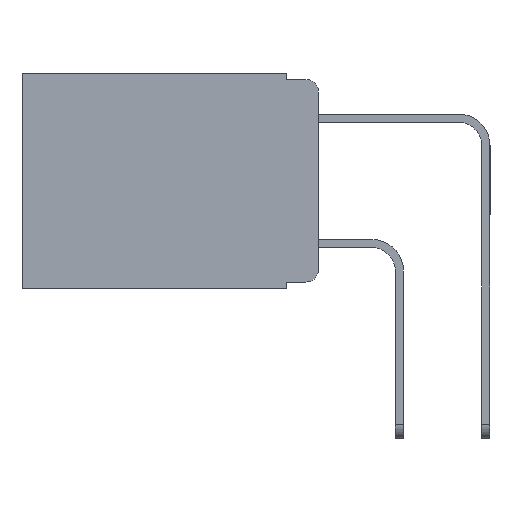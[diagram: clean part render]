
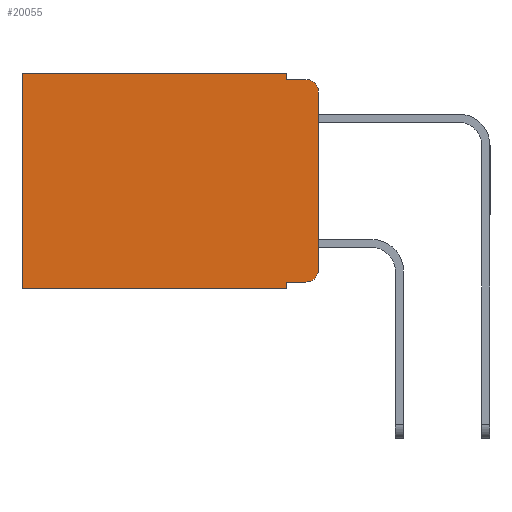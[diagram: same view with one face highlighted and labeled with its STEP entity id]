
A CAD part, left-side view. The second image highlights one B-rep face of the part: STEP entity #20055.
In plain terms, the highlighted planar face has unit normal (-1, 0, 0).
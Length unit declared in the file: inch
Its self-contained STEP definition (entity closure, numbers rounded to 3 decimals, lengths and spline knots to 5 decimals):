
#54 = CARTESIAN_POINT ( 'NONE',  ( 0.298, 0.051, -0.343 ) ) ;
#188 = LINE ( 'NONE', #1957, #16687 ) ;
#774 = AXIS2_PLACEMENT_3D ( 'NONE', #19364, #19434, #10102 ) ;
#894 = LINE ( 'NONE', #9400, #4678 ) ;
#959 = CARTESIAN_POINT ( 'NONE',  ( 0.298, 0.02, -0.313 ) ) ;
#1006 = VERTEX_POINT ( 'NONE', #2538 ) ;
#1144 = CARTESIAN_POINT ( 'NONE',  ( 0.298, 0., -0.03 ) ) ;
#1451 = CARTESIAN_POINT ( 'NONE',  ( 0.298, 0.051, -0.01 ) ) ;
#1523 = LINE ( 'NONE', #11746, #13294 ) ;
#1579 = EDGE_CURVE ( 'NONE', #17158, #1006, #1523, .T. ) ;
#1843 = ORIENTED_EDGE ( 'NONE', *, *, #18049, .F. ) ;
#1889 = LINE ( 'NONE', #14975, #10438 ) ;
#1957 = CARTESIAN_POINT ( 'NONE',  ( 0.298, 0., 0. ) ) ;
#2538 = CARTESIAN_POINT ( 'NONE',  ( 0.298, 0.473, -0.343 ) ) ;
#2570 = DIRECTION ( 'NONE',  ( 0., 0., -1. ) ) ;
#2742 = EDGE_CURVE ( 'NONE', #5668, #14277, #188, .T. ) ;
#3041 = CARTESIAN_POINT ( 'NONE',  ( 0.298, 0.02, -0.333 ) ) ;
#3396 = CARTESIAN_POINT ( 'NONE',  ( 0.298, 0.02, -0.03 ) ) ;
#3581 = CIRCLE ( 'NONE', #18429, 0.02 ) ;
#3601 = CIRCLE ( 'NONE', #11106, 0.02 ) ;
#3774 = VERTEX_POINT ( 'NONE', #10031 ) ;
#3812 = EDGE_CURVE ( 'NONE', #5950, #5194, #19744, .T. ) ;
#3840 = DIRECTION ( 'NONE',  ( 0., -1., 0. ) ) ;
#4229 = LINE ( 'NONE', #10632, #11732 ) ;
#4421 = DIRECTION ( 'NONE',  ( 0., -1., 0. ) ) ;
#4612 = ORIENTED_EDGE ( 'NONE', *, *, #2742, .F. ) ;
#4678 = VECTOR ( 'NONE', #18772, 39.37008 ) ;
#4864 = DIRECTION ( 'NONE',  ( 0., 0., -1. ) ) ;
#5055 = DIRECTION ( 'NONE',  ( 0., 0., -1. ) ) ;
#5194 = VERTEX_POINT ( 'NONE', #1451 ) ;
#5204 = VERTEX_POINT ( 'NONE', #12632 ) ;
#5668 = VERTEX_POINT ( 'NONE', #1144 ) ;
#5950 = VERTEX_POINT ( 'NONE', #6714 ) ;
#6148 = ORIENTED_EDGE ( 'NONE', *, *, #16682, .F. ) ;
#6321 = EDGE_CURVE ( 'NONE', #5194, #3774, #11871, .T. ) ;
#6486 = CARTESIAN_POINT ( 'NONE',  ( 0.298, 0.051, 0. ) ) ;
#6655 = ORIENTED_EDGE ( 'NONE', *, *, #18412, .T. ) ;
#6714 = CARTESIAN_POINT ( 'NONE',  ( 0.298, 0.051, 0. ) ) ;
#7264 = DIRECTION ( 'NONE',  ( 0., 0., -1. ) ) ;
#7406 = VECTOR ( 'NONE', #4864, 39.37008 ) ;
#7438 = CARTESIAN_POINT ( 'NONE',  ( 0.298, 0.473, 0. ) ) ;
#8368 = CARTESIAN_POINT ( 'NONE',  ( 0.298, 0.051, 0. ) ) ;
#8414 = EDGE_CURVE ( 'NONE', #5950, #17158, #4229, .T. ) ;
#8907 = ORIENTED_EDGE ( 'NONE', *, *, #3812, .F. ) ;
#9083 = CARTESIAN_POINT ( 'NONE',  ( 0.298, 0.051, -0.01 ) ) ;
#9105 = CARTESIAN_POINT ( 'NONE',  ( 0.298, 0., -0.313 ) ) ;
#9388 = ORIENTED_EDGE ( 'NONE', *, *, #1579, .T. ) ;
#9400 = CARTESIAN_POINT ( 'NONE',  ( 0.298, 0., -0.343 ) ) ;
#9553 = DIRECTION ( 'NONE',  ( 0., 0., -1. ) ) ;
#10031 = CARTESIAN_POINT ( 'NONE',  ( 0.298, 0.02, -0.01 ) ) ;
#10102 = DIRECTION ( 'NONE',  ( 0., 0., -1. ) ) ;
#10438 = VECTOR ( 'NONE', #3840, 39.37008 ) ;
#10632 = CARTESIAN_POINT ( 'NONE',  ( 0.298, 0., 0. ) ) ;
#10913 = DIRECTION ( 'NONE',  ( 0., 0., -1. ) ) ;
#11031 = EDGE_CURVE ( 'NONE', #5668, #3774, #3601, .T. ) ;
#11106 = AXIS2_PLACEMENT_3D ( 'NONE', #3396, #14552, #5055 ) ;
#11451 = VECTOR ( 'NONE', #7264, 39.37008 ) ;
#11732 = VECTOR ( 'NONE', #19961, 39.37008 ) ;
#11746 = CARTESIAN_POINT ( 'NONE',  ( 0.298, 0.473, 0. ) ) ;
#11871 = LINE ( 'NONE', #9083, #19668 ) ;
#12159 = DIRECTION ( 'NONE',  ( -1., 0., 0. ) ) ;
#12632 = CARTESIAN_POINT ( 'NONE',  ( 0.298, 0.051, -0.333 ) ) ;
#12689 = VERTEX_POINT ( 'NONE', #3041 ) ;
#13111 = ORIENTED_EDGE ( 'NONE', *, *, #6321, .F. ) ;
#13294 = VECTOR ( 'NONE', #9553, 39.37008 ) ;
#13597 = ORIENTED_EDGE ( 'NONE', *, *, #8414, .T. ) ;
#14277 = VERTEX_POINT ( 'NONE', #9105 ) ;
#14552 = DIRECTION ( 'NONE',  ( -1., 0., 0. ) ) ;
#14975 = CARTESIAN_POINT ( 'NONE',  ( 0.298, 0.051, -0.333 ) ) ;
#15788 = EDGE_LOOP ( 'NONE', ( #4612, #16799, #13111, #8907, #13597, #9388, #6148, #1843, #19183, #6655 ) ) ;
#16682 = EDGE_CURVE ( 'NONE', #17426, #1006, #894, .T. ) ;
#16687 = VECTOR ( 'NONE', #10913, 39.37008 ) ;
#16799 = ORIENTED_EDGE ( 'NONE', *, *, #11031, .T. ) ;
#16937 = FACE_OUTER_BOUND ( 'NONE', #15788, .T. ) ;
#17022 = EDGE_CURVE ( 'NONE', #5204, #12689, #1889, .T. ) ;
#17158 = VERTEX_POINT ( 'NONE', #7438 ) ;
#17426 = VERTEX_POINT ( 'NONE', #54 ) ;
#17914 = PLANE ( 'NONE',  #774 ) ;
#18049 = EDGE_CURVE ( 'NONE', #5204, #17426, #20343, .T. ) ;
#18412 = EDGE_CURVE ( 'NONE', #12689, #14277, #3581, .T. ) ;
#18429 = AXIS2_PLACEMENT_3D ( 'NONE', #959, #12159, #2570 ) ;
#18772 = DIRECTION ( 'NONE',  ( 0., 1., 0. ) ) ;
#19183 = ORIENTED_EDGE ( 'NONE', *, *, #17022, .T. ) ;
#19364 = CARTESIAN_POINT ( 'NONE',  ( 0.298, 0., 0. ) ) ;
#19434 = DIRECTION ( 'NONE',  ( 1., 0., 0. ) ) ;
#19668 = VECTOR ( 'NONE', #4421, 39.37008 ) ;
#19744 = LINE ( 'NONE', #8368, #11451 ) ;
#19961 = DIRECTION ( 'NONE',  ( 0., 1., 0. ) ) ;
#20055 = ADVANCED_FACE ( 'NONE', ( #16937 ), #17914, .F. ) ;
#20343 = LINE ( 'NONE', #6486, #7406 ) ;
